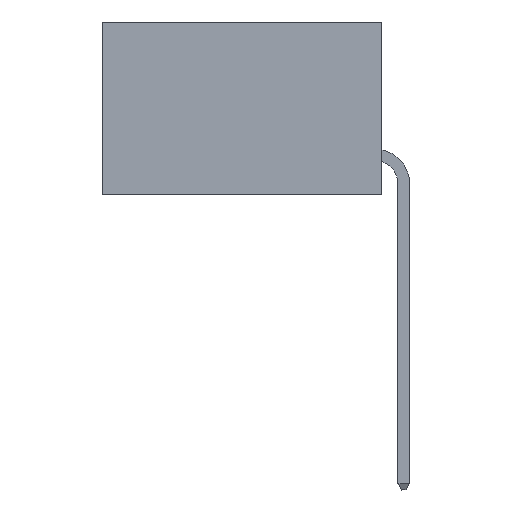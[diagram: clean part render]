
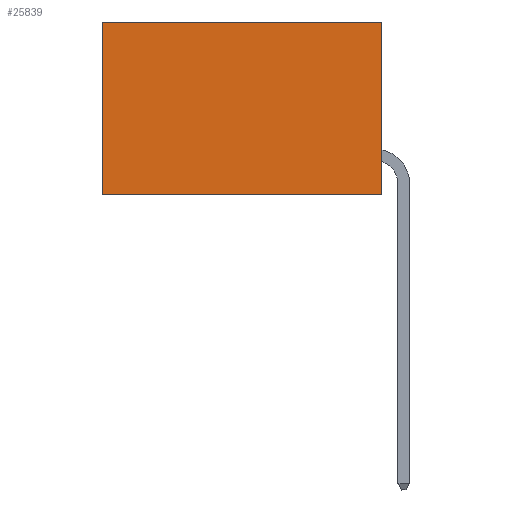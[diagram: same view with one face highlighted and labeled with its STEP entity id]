
A CAD part, left-side view. The second image highlights one B-rep face of the part: STEP entity #25839.
In plain terms, the highlighted planar face has unit normal (-1, 0, 0).
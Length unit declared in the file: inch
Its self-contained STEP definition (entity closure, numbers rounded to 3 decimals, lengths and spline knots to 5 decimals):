
#739 = CARTESIAN_POINT ( 'NONE',  ( 0.2875, 0., 0. ) ) ;
#2945 = VECTOR ( 'NONE', #24727, 39.37008 ) ;
#5699 = CARTESIAN_POINT ( 'NONE',  ( 0.2875, 0.6, -0.37 ) ) ;
#7298 = DIRECTION ( 'NONE',  ( 0., 1., 0. ) ) ;
#8421 = VECTOR ( 'NONE', #16346, 39.37008 ) ;
#12112 = ORIENTED_EDGE ( 'NONE', *, *, #31074, .T. ) ;
#12868 = LINE ( 'NONE', #20939, #2945 ) ;
#13321 = CARTESIAN_POINT ( 'NONE',  ( 0.2875, 0.6, 0. ) ) ;
#16346 = DIRECTION ( 'NONE',  ( 0., 1., 0. ) ) ;
#17634 = FACE_OUTER_BOUND ( 'NONE', #36008, .T. ) ;
#20217 = VERTEX_POINT ( 'NONE', #21959 ) ;
#20725 = DIRECTION ( 'NONE',  ( 0., 0., -1. ) ) ;
#20939 = CARTESIAN_POINT ( 'NONE',  ( 0.2875, 0., 0. ) ) ;
#21959 = CARTESIAN_POINT ( 'NONE',  ( 0.2875, 0., 0. ) ) ;
#22899 = CARTESIAN_POINT ( 'NONE',  ( 0.2875, 0., 0. ) ) ;
#23281 = CARTESIAN_POINT ( 'NONE',  ( 0.2875, 0., -0.37 ) ) ;
#24727 = DIRECTION ( 'NONE',  ( 0., 0., -1. ) ) ;
#25839 = ADVANCED_FACE ( 'NONE', ( #17634 ), #45765, .F. ) ;
#26258 = ORIENTED_EDGE ( 'NONE', *, *, #30248, .F. ) ;
#27679 = EDGE_CURVE ( 'NONE', #20217, #34087, #36042, .T. ) ;
#28275 = ORIENTED_EDGE ( 'NONE', *, *, #45382, .F. ) ;
#28733 = LINE ( 'NONE', #13321, #29930 ) ;
#29930 = VECTOR ( 'NONE', #20725, 39.37008 ) ;
#30248 = EDGE_CURVE ( 'NONE', #20217, #33582, #12868, .T. ) ;
#31074 = EDGE_CURVE ( 'NONE', #34087, #42967, #28733, .T. ) ;
#31318 = ORIENTED_EDGE ( 'NONE', *, *, #27679, .T. ) ;
#31741 = AXIS2_PLACEMENT_3D ( 'NONE', #739, #38700, #46236 ) ;
#32071 = CARTESIAN_POINT ( 'NONE',  ( 0.2875, 0.6, 0. ) ) ;
#33582 = VERTEX_POINT ( 'NONE', #40708 ) ;
#34087 = VERTEX_POINT ( 'NONE', #32071 ) ;
#36008 = EDGE_LOOP ( 'NONE', ( #12112, #28275, #26258, #31318 ) ) ;
#36042 = LINE ( 'NONE', #22899, #39605 ) ;
#38700 = DIRECTION ( 'NONE',  ( 1., 0., 0. ) ) ;
#39605 = VECTOR ( 'NONE', #7298, 39.37008 ) ;
#40708 = CARTESIAN_POINT ( 'NONE',  ( 0.2875, 0., -0.37 ) ) ;
#42967 = VERTEX_POINT ( 'NONE', #5699 ) ;
#43151 = LINE ( 'NONE', #23281, #8421 ) ;
#45382 = EDGE_CURVE ( 'NONE', #33582, #42967, #43151, .T. ) ;
#45765 = PLANE ( 'NONE',  #31741 ) ;
#46236 = DIRECTION ( 'NONE',  ( 0., 0., -1. ) ) ;
